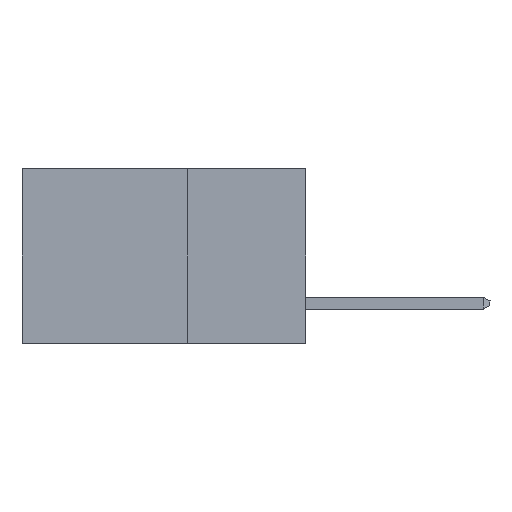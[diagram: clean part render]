
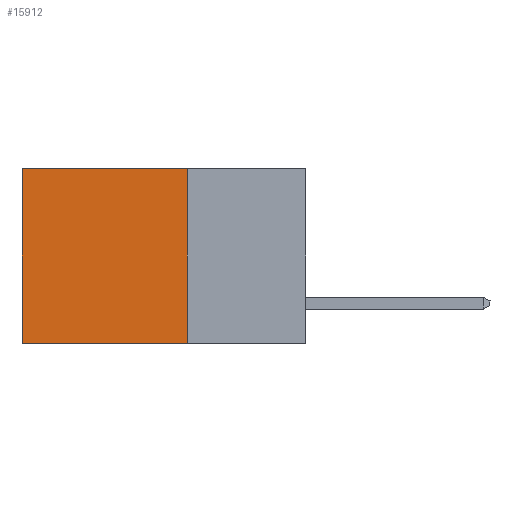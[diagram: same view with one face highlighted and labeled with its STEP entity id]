
A CAD part, left-side view. The second image highlights one B-rep face of the part: STEP entity #15912.
In plain terms, the highlighted planar face has unit normal (-1, 0, 0).
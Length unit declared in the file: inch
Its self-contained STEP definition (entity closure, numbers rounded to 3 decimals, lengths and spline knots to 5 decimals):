
#274 = VERTEX_POINT ( 'NONE', #18119 ) ;
#388 = DIRECTION ( 'NONE',  ( 0., 0., -1. ) ) ;
#467 = CARTESIAN_POINT ( 'NONE',  ( 0.298, 0.25, 0. ) ) ;
#920 = VECTOR ( 'NONE', #15825, 39.37008 ) ;
#1193 = ORIENTED_EDGE ( 'NONE', *, *, #1401, .T. ) ;
#1401 = EDGE_CURVE ( 'NONE', #12182, #274, #10967, .T. ) ;
#2060 = LINE ( 'NONE', #19133, #16560 ) ;
#2067 = CARTESIAN_POINT ( 'NONE',  ( 0.298, 0.25, 0. ) ) ;
#2312 = DIRECTION ( 'NONE',  ( 1., 0., 0. ) ) ;
#2889 = AXIS2_PLACEMENT_3D ( 'NONE', #467, #2312, #388 ) ;
#3113 = EDGE_CURVE ( 'NONE', #6701, #17469, #19741, .T. ) ;
#3774 = DIRECTION ( 'NONE',  ( 0., 1., 0. ) ) ;
#6284 = VECTOR ( 'NONE', #7127, 39.37008 ) ;
#6476 = LINE ( 'NONE', #17641, #20448 ) ;
#6691 = ORIENTED_EDGE ( 'NONE', *, *, #9848, .F. ) ;
#6701 = VERTEX_POINT ( 'NONE', #11946 ) ;
#6969 = CARTESIAN_POINT ( 'NONE',  ( 0.298, 0.25, -0.37 ) ) ;
#7127 = DIRECTION ( 'NONE',  ( 0., 0., -1. ) ) ;
#8163 = ORIENTED_EDGE ( 'NONE', *, *, #3113, .F. ) ;
#8994 = PLANE ( 'NONE',  #2889 ) ;
#9848 = EDGE_CURVE ( 'NONE', #17469, #274, #6476, .T. ) ;
#10627 = CARTESIAN_POINT ( 'NONE',  ( 0.298, 0.6, 0. ) ) ;
#10967 = LINE ( 'NONE', #10627, #6284 ) ;
#11593 = CARTESIAN_POINT ( 'NONE',  ( 0.298, 0.6, 0. ) ) ;
#11946 = CARTESIAN_POINT ( 'NONE',  ( 0.298, 0.25, 0. ) ) ;
#12182 = VERTEX_POINT ( 'NONE', #11593 ) ;
#15716 = DIRECTION ( 'NONE',  ( 0., 1., 0. ) ) ;
#15825 = DIRECTION ( 'NONE',  ( 0., 0., -1. ) ) ;
#15912 = ADVANCED_FACE ( 'NONE', ( #16281 ), #8994, .F. ) ;
#16281 = FACE_OUTER_BOUND ( 'NONE', #18692, .T. ) ;
#16373 = ORIENTED_EDGE ( 'NONE', *, *, #19264, .T. ) ;
#16560 = VECTOR ( 'NONE', #15716, 39.37008 ) ;
#17469 = VERTEX_POINT ( 'NONE', #6969 ) ;
#17641 = CARTESIAN_POINT ( 'NONE',  ( 0.298, 0.25, -0.37 ) ) ;
#18119 = CARTESIAN_POINT ( 'NONE',  ( 0.298, 0.6, -0.37 ) ) ;
#18692 = EDGE_LOOP ( 'NONE', ( #1193, #6691, #8163, #16373 ) ) ;
#19133 = CARTESIAN_POINT ( 'NONE',  ( 0.298, 0.25, 0. ) ) ;
#19264 = EDGE_CURVE ( 'NONE', #6701, #12182, #2060, .T. ) ;
#19741 = LINE ( 'NONE', #2067, #920 ) ;
#20448 = VECTOR ( 'NONE', #3774, 39.37008 ) ;
